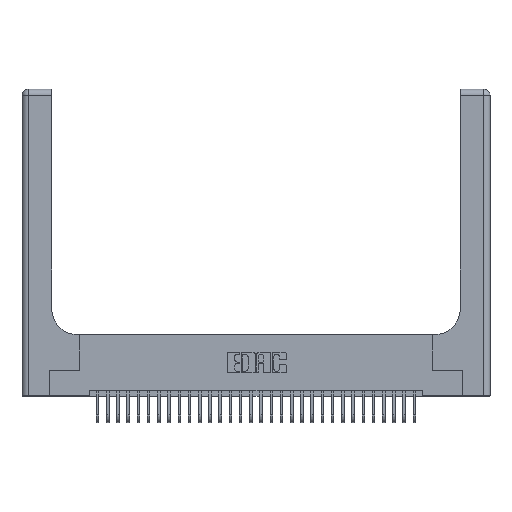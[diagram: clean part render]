
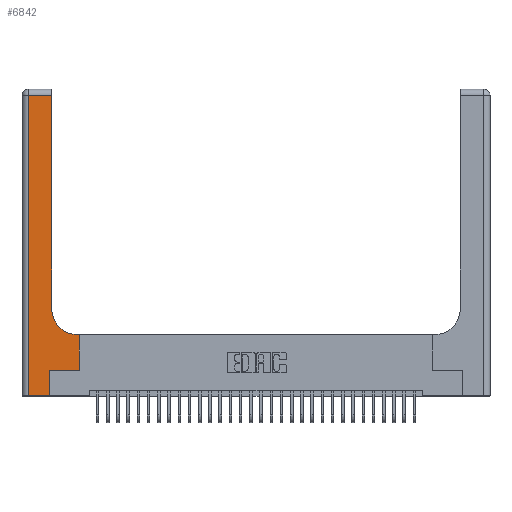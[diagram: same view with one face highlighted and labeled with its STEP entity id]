
A CAD part, top view. The second image highlights one B-rep face of the part: STEP entity #6842.
In plain terms, the highlighted planar face has unit normal (0, 0, 1).
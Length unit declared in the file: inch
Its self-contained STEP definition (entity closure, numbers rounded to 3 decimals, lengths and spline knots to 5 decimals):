
#1435 = ORIENTED_EDGE ( 'NONE', *, *, #16743, .T. ) ;
#1500 = LINE ( 'NONE', #30762, #17202 ) ;
#1863 = EDGE_CURVE ( 'NONE', #10761, #4932, #28157, .T. ) ;
#2024 = CARTESIAN_POINT ( 'NONE',  ( 0.06, 2.94, 0.37 ) ) ;
#3417 = AXIS2_PLACEMENT_3D ( 'NONE', #20109, #22672, #28072 ) ;
#3671 = ORIENTED_EDGE ( 'NONE', *, *, #27197, .T. ) ;
#4033 = DIRECTION ( 'NONE',  ( 0., 1., 0. ) ) ;
#4426 = VECTOR ( 'NONE', #4033, 39.37008 ) ;
#4932 = VERTEX_POINT ( 'NONE', #22879 ) ;
#5762 = LINE ( 'NONE', #16351, #26250 ) ;
#5973 = EDGE_CURVE ( 'NONE', #26589, #11636, #30576, .T. ) ;
#6842 = ADVANCED_FACE ( 'NONE', ( #20460 ), #31535, .F. ) ;
#7134 = CARTESIAN_POINT ( 'NONE',  ( 0.5415, 0.6, 0.37 ) ) ;
#8461 = ORIENTED_EDGE ( 'NONE', *, *, #17123, .T. ) ;
#8629 = DIRECTION ( 'NONE',  ( 0., 0., -1. ) ) ;
#8638 = DIRECTION ( 'NONE',  ( 0., 1., 0. ) ) ;
#9058 = ORIENTED_EDGE ( 'NONE', *, *, #21119, .T. ) ;
#9364 = CARTESIAN_POINT ( 'NONE',  ( 0.2915, 3., 0.37 ) ) ;
#10326 = CARTESIAN_POINT ( 'NONE',  ( 0.269, 0., 0.37 ) ) ;
#10761 = VERTEX_POINT ( 'NONE', #12063 ) ;
#11474 = DIRECTION ( 'NONE',  ( 0., 1., 0. ) ) ;
#11487 = CARTESIAN_POINT ( 'NONE',  ( 0.06, 0., 0.37 ) ) ;
#11636 = VERTEX_POINT ( 'NONE', #22032 ) ;
#12063 = CARTESIAN_POINT ( 'NONE',  ( 0.2915, 0.85, 0.37 ) ) ;
#12789 = DIRECTION ( 'NONE',  ( -1., 0., 0. ) ) ;
#13003 = DIRECTION ( 'NONE',  ( 1., 0., 0. ) ) ;
#13656 = DIRECTION ( 'NONE',  ( -1., 0., 0. ) ) ;
#13676 = CARTESIAN_POINT ( 'NONE',  ( 0.269, 0., 0.37 ) ) ;
#16351 = CARTESIAN_POINT ( 'NONE',  ( 0., 2.94, 0.37 ) ) ;
#16450 = LINE ( 'NONE', #10326, #28107 ) ;
#16743 = EDGE_CURVE ( 'NONE', #11636, #29156, #24948, .T. ) ;
#17123 = EDGE_CURVE ( 'NONE', #29156, #10761, #20491, .T. ) ;
#17202 = VECTOR ( 'NONE', #13003, 39.37008 ) ;
#18005 = VERTEX_POINT ( 'NONE', #13676 ) ;
#18061 = EDGE_CURVE ( 'NONE', #18005, #32322, #16450, .T. ) ;
#18503 = ORIENTED_EDGE ( 'NONE', *, *, #1863, .T. ) ;
#20109 = CARTESIAN_POINT ( 'NONE',  ( 0.5415, 0.85, 0.37 ) ) ;
#20118 = VECTOR ( 'NONE', #11474, 39.37008 ) ;
#20203 = CARTESIAN_POINT ( 'NONE',  ( 0.5585, 0.25, 0.37 ) ) ;
#20460 = FACE_OUTER_BOUND ( 'NONE', #22570, .T. ) ;
#20491 = CIRCLE ( 'NONE', #3417, 0.25 ) ;
#20701 = ORIENTED_EDGE ( 'NONE', *, *, #32293, .T. ) ;
#21119 = EDGE_CURVE ( 'NONE', #4932, #27662, #5762, .T. ) ;
#21984 = AXIS2_PLACEMENT_3D ( 'NONE', #29026, #8629, #13656 ) ;
#22017 = LINE ( 'NONE', #30247, #31298 ) ;
#22032 = CARTESIAN_POINT ( 'NONE',  ( 0.5585, 0.6, 0.37 ) ) ;
#22570 = EDGE_LOOP ( 'NONE', ( #18503, #9058, #32715, #3671, #32845, #20701, #23189, #1435, #8461 ) ) ;
#22672 = DIRECTION ( 'NONE',  ( 0., 0., -1. ) ) ;
#22879 = CARTESIAN_POINT ( 'NONE',  ( 0.2915, 2.94, 0.37 ) ) ;
#23039 = VECTOR ( 'NONE', #32555, 39.37008 ) ;
#23094 = CARTESIAN_POINT ( 'NONE',  ( 0.269, 0.25, 0.37 ) ) ;
#23189 = ORIENTED_EDGE ( 'NONE', *, *, #5973, .T. ) ;
#24602 = CARTESIAN_POINT ( 'NONE',  ( 0.5585, 0.25, 0.37 ) ) ;
#24948 = LINE ( 'NONE', #28920, #31371 ) ;
#25457 = LINE ( 'NONE', #27098, #23039 ) ;
#26250 = VECTOR ( 'NONE', #31978, 39.37008 ) ;
#26589 = VERTEX_POINT ( 'NONE', #20203 ) ;
#27098 = CARTESIAN_POINT ( 'NONE',  ( 0., 0., 0.37 ) ) ;
#27197 = EDGE_CURVE ( 'NONE', #30722, #18005, #25457, .T. ) ;
#27662 = VERTEX_POINT ( 'NONE', #2024 ) ;
#28072 = DIRECTION ( 'NONE',  ( 1., 0., 0. ) ) ;
#28107 = VECTOR ( 'NONE', #8638, 39.37008 ) ;
#28157 = LINE ( 'NONE', #9364, #4426 ) ;
#28920 = CARTESIAN_POINT ( 'NONE',  ( 0.2915, 0.6, 0.37 ) ) ;
#29026 = CARTESIAN_POINT ( 'NONE',  ( 0., 3., 0.37 ) ) ;
#29156 = VERTEX_POINT ( 'NONE', #7134 ) ;
#30247 = CARTESIAN_POINT ( 'NONE',  ( 0.06, 3., 0.37 ) ) ;
#30576 = LINE ( 'NONE', #24602, #20118 ) ;
#30722 = VERTEX_POINT ( 'NONE', #11487 ) ;
#30762 = CARTESIAN_POINT ( 'NONE',  ( 0.269, 0.25, 0.37 ) ) ;
#31298 = VECTOR ( 'NONE', #32754, 39.37008 ) ;
#31371 = VECTOR ( 'NONE', #12789, 39.37008 ) ;
#31535 = PLANE ( 'NONE',  #21984 ) ;
#31557 = EDGE_CURVE ( 'NONE', #27662, #30722, #22017, .T. ) ;
#31978 = DIRECTION ( 'NONE',  ( -1., 0., 0. ) ) ;
#32293 = EDGE_CURVE ( 'NONE', #32322, #26589, #1500, .T. ) ;
#32322 = VERTEX_POINT ( 'NONE', #23094 ) ;
#32555 = DIRECTION ( 'NONE',  ( 1., 0., 0. ) ) ;
#32715 = ORIENTED_EDGE ( 'NONE', *, *, #31557, .T. ) ;
#32754 = DIRECTION ( 'NONE',  ( 0., -1., 0. ) ) ;
#32845 = ORIENTED_EDGE ( 'NONE', *, *, #18061, .T. ) ;
